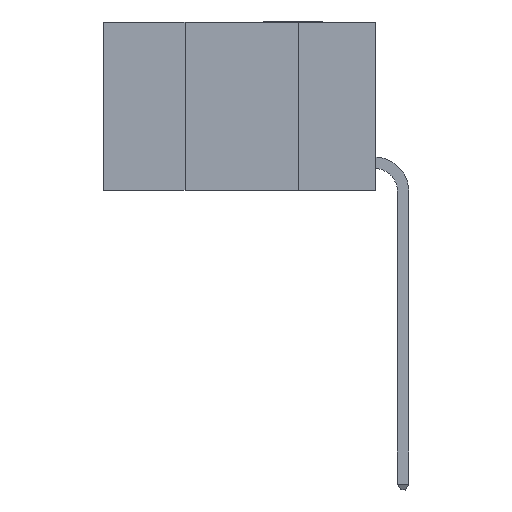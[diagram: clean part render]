
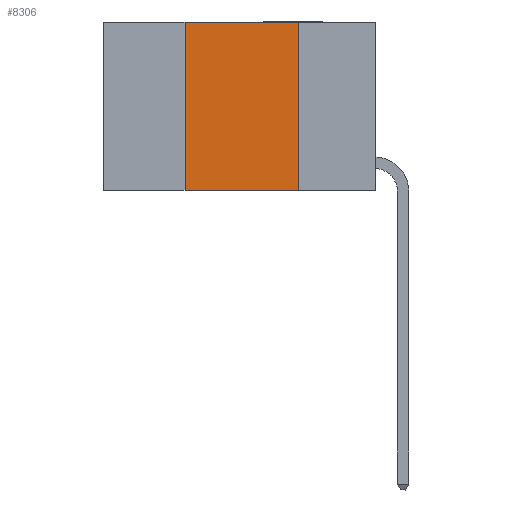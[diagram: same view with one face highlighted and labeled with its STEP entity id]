
A CAD part, left-side view. The second image highlights one B-rep face of the part: STEP entity #8306.
In plain terms, the highlighted planar face has unit normal (-1, 0, 0).
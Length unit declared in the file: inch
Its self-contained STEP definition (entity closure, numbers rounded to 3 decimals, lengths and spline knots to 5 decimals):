
#141 = CARTESIAN_POINT ( 'NONE',  ( 0., 0.6, 0. ) ) ;
#176 = DIRECTION ( 'NONE',  ( 0., 0., -1. ) ) ;
#401 = DIRECTION ( 'NONE',  ( 0., 0., 1. ) ) ;
#759 = LINE ( 'NONE', #2677, #4400 ) ;
#788 = VECTOR ( 'NONE', #3038, 39.37008 ) ;
#1267 = LINE ( 'NONE', #4342, #788 ) ;
#1690 = CARTESIAN_POINT ( 'NONE',  ( 0., 0.17, 0. ) ) ;
#1815 = ORIENTED_EDGE ( 'NONE', *, *, #5940, .T. ) ;
#2018 = EDGE_LOOP ( 'NONE', ( #8196, #5737, #4310, #1815 ) ) ;
#2093 = CARTESIAN_POINT ( 'NONE',  ( 0., 0.42, 0. ) ) ;
#2367 = PLANE ( 'NONE',  #6162 ) ;
#2435 = CARTESIAN_POINT ( 'NONE',  ( 0., 0.17, -0.37 ) ) ;
#2600 = DIRECTION ( 'NONE',  ( 0., -1., 0. ) ) ;
#2677 = CARTESIAN_POINT ( 'NONE',  ( 0., 0.42, 0. ) ) ;
#3038 = DIRECTION ( 'NONE',  ( 0., -1., 0. ) ) ;
#3114 = EDGE_CURVE ( 'NONE', #6844, #3723, #759, .T. ) ;
#3488 = CARTESIAN_POINT ( 'NONE',  ( 0., 0.17, 0. ) ) ;
#3723 = VERTEX_POINT ( 'NONE', #2093 ) ;
#3990 = EDGE_CURVE ( 'NONE', #4898, #5034, #7715, .T. ) ;
#4310 = ORIENTED_EDGE ( 'NONE', *, *, #3114, .F. ) ;
#4342 = CARTESIAN_POINT ( 'NONE',  ( 0., 0.6, 0. ) ) ;
#4359 = DIRECTION ( 'NONE',  ( 1., 0., 0. ) ) ;
#4400 = VECTOR ( 'NONE', #401, 39.37008 ) ;
#4898 = VERTEX_POINT ( 'NONE', #3488 ) ;
#5034 = VERTEX_POINT ( 'NONE', #2435 ) ;
#5447 = FACE_OUTER_BOUND ( 'NONE', #2018, .T. ) ;
#5549 = DIRECTION ( 'NONE',  ( 0., 0., -1. ) ) ;
#5737 = ORIENTED_EDGE ( 'NONE', *, *, #7770, .F. ) ;
#5750 = CARTESIAN_POINT ( 'NONE',  ( 0., 0.6, -0.37 ) ) ;
#5865 = LINE ( 'NONE', #5750, #7422 ) ;
#5940 = EDGE_CURVE ( 'NONE', #6844, #5034, #5865, .T. ) ;
#6162 = AXIS2_PLACEMENT_3D ( 'NONE', #141, #4359, #176 ) ;
#6343 = VECTOR ( 'NONE', #5549, 39.37008 ) ;
#6844 = VERTEX_POINT ( 'NONE', #7001 ) ;
#7001 = CARTESIAN_POINT ( 'NONE',  ( 0., 0.42, -0.37 ) ) ;
#7422 = VECTOR ( 'NONE', #2600, 39.37008 ) ;
#7715 = LINE ( 'NONE', #1690, #6343 ) ;
#7770 = EDGE_CURVE ( 'NONE', #3723, #4898, #1267, .T. ) ;
#8196 = ORIENTED_EDGE ( 'NONE', *, *, #3990, .F. ) ;
#8306 = ADVANCED_FACE ( 'NONE', ( #5447 ), #2367, .F. ) ;
